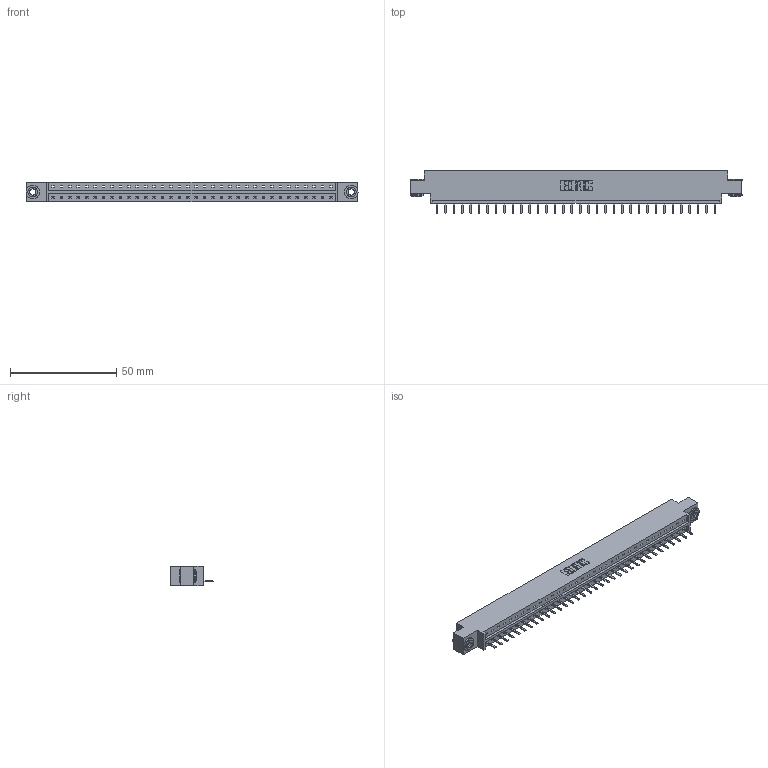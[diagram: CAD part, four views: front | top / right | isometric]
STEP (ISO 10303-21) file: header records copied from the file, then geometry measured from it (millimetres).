
FILE_DESCRIPTION (( 'STEP AP203' ), '1' );
FILE_NAME ('833-034-520-603.STEP', '2020-06-02T21:18:17', ( '' ), ( '' ), 'SwSTEP 2.0', 'SolidWorks 2020', '' );
FILE_SCHEMA (( 'CONFIG_CONTROL_DESIGN' ));
Length unit declared in the file: inch
Products named in the file (4): 345-250-002_345-250-002-102; 833 Part_Offset - .156 Dia - TH; 833-034-520-603; 345-292-001_345-293-120
Assembly tree (37 placements, depth 2):
  833-034-520-603
    833 Part_Offset - .156 Dia - TH
    345-292-001_345-293-120  x34
    345-250-002_345-250-002-102  x2
Bounding box: 156.26 x 20.02 x 9.4 mm (x, y, z)
Volume: 15349.2 mm3; surface area: 16637.8 mm2
Topology: 37 solids, 37 shells, 2264 faces, 6655 edges, 4342 vertices
Faces by surface type: plane 1580, cylinder 676, cone 8
Entity records: 22716 total; most frequent: CARTESIAN_POINT 3911, ORIENTED_EDGE 3862, DIRECTION 3337, EDGE_CURVE 1931, VECTOR 1775, LINE 1775, VERTEX_POINT 1282, AXIS2_PLACEMENT_3D 781
